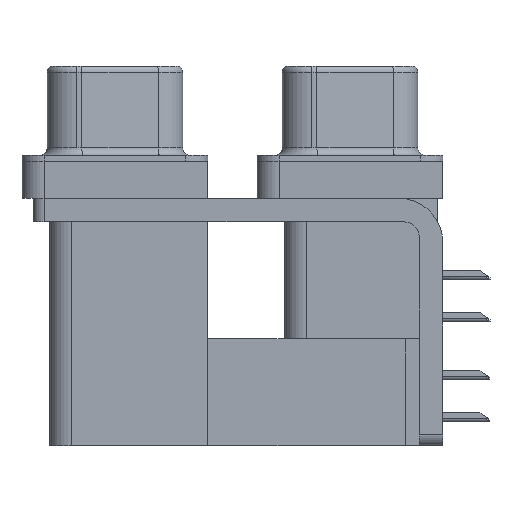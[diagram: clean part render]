
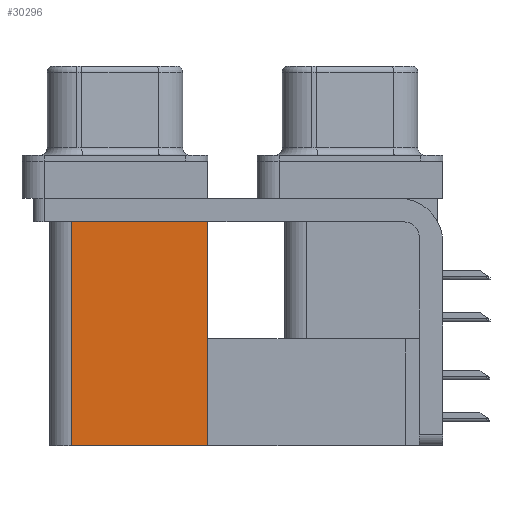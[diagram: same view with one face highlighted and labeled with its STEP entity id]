
A CAD part, left-side view. The second image highlights one B-rep face of the part: STEP entity #30296.
In plain terms, the highlighted planar face has unit normal (-1, 0, 0).
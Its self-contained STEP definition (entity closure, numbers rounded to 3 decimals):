
#959 = VERTEX_POINT ( 'NONE', #30878 ) ;
#2468 = VERTEX_POINT ( 'NONE', #5191 ) ;
#3154 = CARTESIAN_POINT ( 'NONE',  ( 3.765, 9.6, -19.2 ) ) ;
#4191 = CARTESIAN_POINT ( 'NONE',  ( 3.765, 18.8, -19.2 ) ) ;
#4238 = EDGE_CURVE ( 'NONE', #7579, #959, #9743, .T. ) ;
#5191 = CARTESIAN_POINT ( 'NONE',  ( 3.765, 9.6, -2.5 ) ) ;
#5614 = CARTESIAN_POINT ( 'NONE',  ( 3.765, 18.8, -19.2 ) ) ;
#7346 = VECTOR ( 'NONE', #15807, 1000. ) ;
#7579 = VERTEX_POINT ( 'NONE', #4191 ) ;
#7999 = DIRECTION ( 'NONE',  ( 0., 1., 0. ) ) ;
#8699 = ORIENTED_EDGE ( 'NONE', *, *, #4238, .F. ) ;
#9743 = LINE ( 'NONE', #5614, #23556 ) ;
#10152 = AXIS2_PLACEMENT_3D ( 'NONE', #21612, #28121, #30989 ) ;
#14283 = EDGE_CURVE ( 'NONE', #2468, #959, #29725, .T. ) ;
#15200 = LINE ( 'NONE', #20115, #23191 ) ;
#15266 = DIRECTION ( 'NONE',  ( 0., 0., 1. ) ) ;
#15807 = DIRECTION ( 'NONE',  ( 0., 0., 1. ) ) ;
#16710 = ORIENTED_EDGE ( 'NONE', *, *, #27761, .F. ) ;
#17729 = DIRECTION ( 'NONE',  ( 0., 1., 0. ) ) ;
#18567 = ORIENTED_EDGE ( 'NONE', *, *, #24660, .T. ) ;
#20115 = CARTESIAN_POINT ( 'NONE',  ( 3.765, 9.6, -19.2 ) ) ;
#20343 = CARTESIAN_POINT ( 'NONE',  ( 3.765, 9.6, -2.5 ) ) ;
#21612 = CARTESIAN_POINT ( 'NONE',  ( 3.765, 9.6, -19.2 ) ) ;
#21965 = VECTOR ( 'NONE', #7999, 1000. ) ;
#23191 = VECTOR ( 'NONE', #17729, 1000. ) ;
#23523 = FACE_OUTER_BOUND ( 'NONE', #30103, .T. ) ;
#23556 = VECTOR ( 'NONE', #15266, 1000. ) ;
#23947 = ORIENTED_EDGE ( 'NONE', *, *, #14283, .T. ) ;
#24660 = EDGE_CURVE ( 'NONE', #27426, #2468, #24868, .T. ) ;
#24868 = LINE ( 'NONE', #3154, #7346 ) ;
#27426 = VERTEX_POINT ( 'NONE', #27902 ) ;
#27761 = EDGE_CURVE ( 'NONE', #27426, #7579, #15200, .T. ) ;
#27902 = CARTESIAN_POINT ( 'NONE',  ( 3.765, 9.6, -19.2 ) ) ;
#28121 = DIRECTION ( 'NONE',  ( 1., 0., 0. ) ) ;
#28600 = PLANE ( 'NONE',  #10152 ) ;
#29725 = LINE ( 'NONE', #20343, #21965 ) ;
#30103 = EDGE_LOOP ( 'NONE', ( #23947, #8699, #16710, #18567 ) ) ;
#30296 = ADVANCED_FACE ( 'NONE', ( #23523 ), #28600, .F. ) ;
#30878 = CARTESIAN_POINT ( 'NONE',  ( 3.765, 18.8, -2.5 ) ) ;
#30989 = DIRECTION ( 'NONE',  ( 0., 0., -1. ) ) ;
